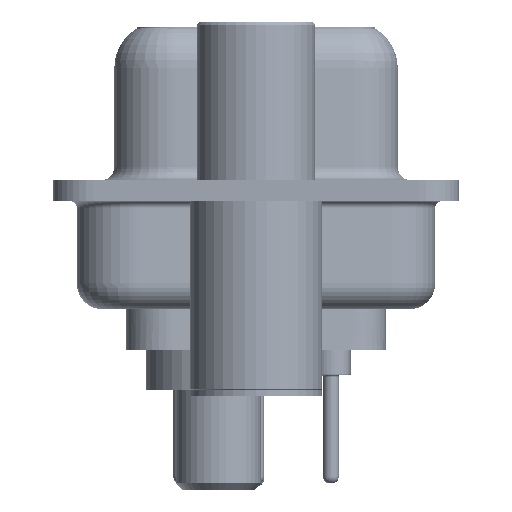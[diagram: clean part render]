
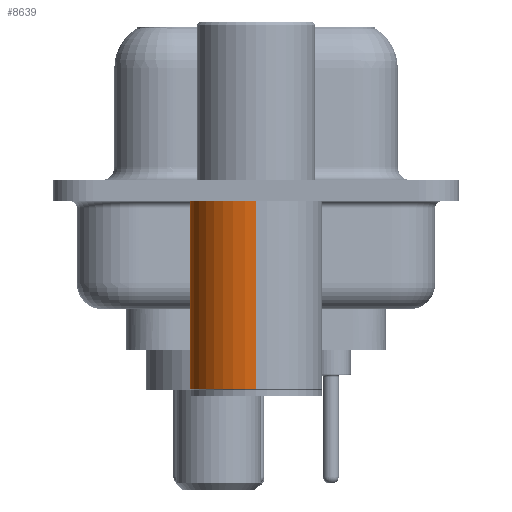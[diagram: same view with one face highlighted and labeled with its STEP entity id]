
A CAD part, left-side view. The second image highlights one B-rep face of the part: STEP entity #8639.
In plain terms, the highlighted cylindrical face has radius 2.5 mm (diameter 5 mm), a partial arc.
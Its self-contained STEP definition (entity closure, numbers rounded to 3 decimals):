
#1172 = CARTESIAN_POINT ( 'NONE',  ( 0., 0., -0.4 ) ) ;
#1761 = EDGE_LOOP ( 'NONE', ( #16407, #28682, #20394, #36311 ) ) ;
#3114 = VERTEX_POINT ( 'NONE', #11287 ) ;
#4707 = DIRECTION ( 'NONE',  ( 0., 0., 1. ) ) ;
#4906 = DIRECTION ( 'NONE',  ( 1., 0., 0. ) ) ;
#6960 = DIRECTION ( 'NONE',  ( 0., 0., 1. ) ) ;
#7425 = CARTESIAN_POINT ( 'NONE',  ( 0., 0., 0.581 ) ) ;
#7770 = CARTESIAN_POINT ( 'NONE',  ( -2.5, 0., -7.525 ) ) ;
#7976 = DIRECTION ( 'NONE',  ( 0., 0., 1. ) ) ;
#8639 = ADVANCED_FACE ( 'NONE', ( #27326 ), #29075, .T. ) ;
#9225 = EDGE_CURVE ( 'NONE', #16991, #3114, #25553, .T. ) ;
#11287 = CARTESIAN_POINT ( 'NONE',  ( 2.5, 0., -0.4 ) ) ;
#12298 = CIRCLE ( 'NONE', #35806, 2.5 ) ;
#13125 = DIRECTION ( 'NONE',  ( 0., 0., 1. ) ) ;
#13514 = AXIS2_PLACEMENT_3D ( 'NONE', #7425, #4707, #18303 ) ;
#16407 = ORIENTED_EDGE ( 'NONE', *, *, #31993, .T. ) ;
#16991 = VERTEX_POINT ( 'NONE', #23559 ) ;
#17719 = LINE ( 'NONE', #24498, #25181 ) ;
#18303 = DIRECTION ( 'NONE',  ( 1., 0., 0. ) ) ;
#19419 = VECTOR ( 'NONE', #7976, 1000. ) ;
#20394 = ORIENTED_EDGE ( 'NONE', *, *, #27743, .F. ) ;
#22246 = VERTEX_POINT ( 'NONE', #27519 ) ;
#22478 = AXIS2_PLACEMENT_3D ( 'NONE', #1172, #6960, #34673 ) ;
#23559 = CARTESIAN_POINT ( 'NONE',  ( 2.5, 0., -7.525 ) ) ;
#24498 = CARTESIAN_POINT ( 'NONE',  ( -2.5, 0., 0.581 ) ) ;
#25181 = VECTOR ( 'NONE', #33085, 1000. ) ;
#25553 = LINE ( 'NONE', #32991, #19419 ) ;
#27326 = FACE_OUTER_BOUND ( 'NONE', #1761, .T. ) ;
#27519 = CARTESIAN_POINT ( 'NONE',  ( -2.5, 0., -0.4 ) ) ;
#27743 = EDGE_CURVE ( 'NONE', #3114, #22246, #27850, .T. ) ;
#27850 = CIRCLE ( 'NONE', #22478, 2.5 ) ;
#28506 = VERTEX_POINT ( 'NONE', #7770 ) ;
#28682 = ORIENTED_EDGE ( 'NONE', *, *, #35927, .T. ) ;
#29075 = CYLINDRICAL_SURFACE ( 'NONE', #13514, 2.5 ) ;
#30274 = CARTESIAN_POINT ( 'NONE',  ( 0., 0., -7.525 ) ) ;
#31993 = EDGE_CURVE ( 'NONE', #16991, #28506, #12298, .T. ) ;
#32991 = CARTESIAN_POINT ( 'NONE',  ( 2.5, 0., 0.581 ) ) ;
#33085 = DIRECTION ( 'NONE',  ( 0., 0., 1. ) ) ;
#34673 = DIRECTION ( 'NONE',  ( 1., 0., 0. ) ) ;
#35806 = AXIS2_PLACEMENT_3D ( 'NONE', #30274, #13125, #4906 ) ;
#35927 = EDGE_CURVE ( 'NONE', #28506, #22246, #17719, .T. ) ;
#36311 = ORIENTED_EDGE ( 'NONE', *, *, #9225, .F. ) ;
